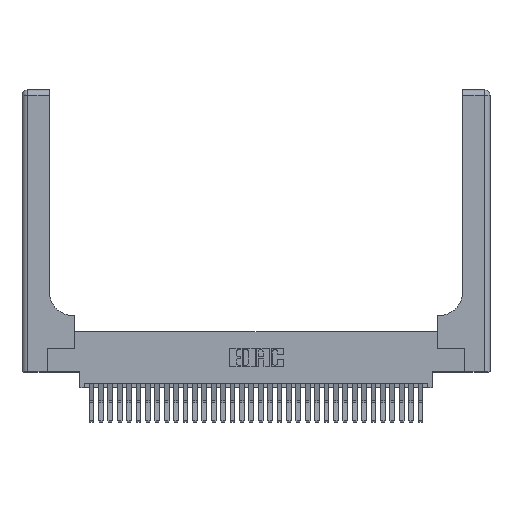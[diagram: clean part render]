
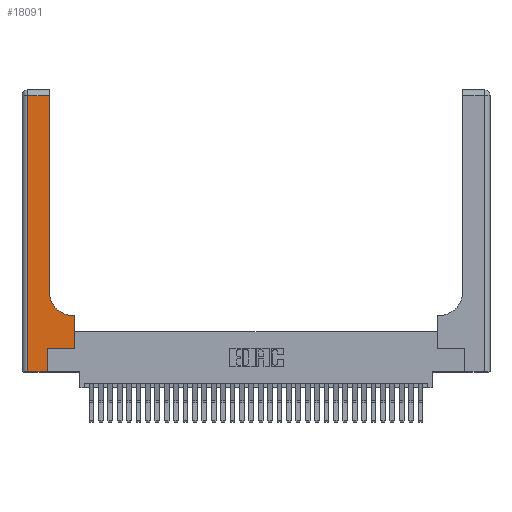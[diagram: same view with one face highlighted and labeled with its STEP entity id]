
A CAD part, top view. The second image highlights one B-rep face of the part: STEP entity #18091.
In plain terms, the highlighted planar face has unit normal (0, 0, 1).
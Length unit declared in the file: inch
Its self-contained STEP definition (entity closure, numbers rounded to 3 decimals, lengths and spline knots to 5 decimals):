
#297 = LINE ( 'NONE', #17229, #12011 ) ;
#355 = LINE ( 'NONE', #4672, #33741 ) ;
#664 = LINE ( 'NONE', #33118, #32364 ) ;
#1186 = VECTOR ( 'NONE', #3302, 39.37008 ) ;
#1492 = DIRECTION ( 'NONE',  ( 0., 1., 0. ) ) ;
#2747 = CARTESIAN_POINT ( 'NONE',  ( 0.2915, 0.6, 0.37 ) ) ;
#2825 = DIRECTION ( 'NONE',  ( -1., 0., 0. ) ) ;
#3302 = DIRECTION ( 'NONE',  ( 1., 0., 0. ) ) ;
#3813 = ORIENTED_EDGE ( 'NONE', *, *, #15643, .T. ) ;
#4265 = DIRECTION ( 'NONE',  ( 0., 1., 0. ) ) ;
#4672 = CARTESIAN_POINT ( 'NONE',  ( 0., 2.94, 0.37 ) ) ;
#4776 = CARTESIAN_POINT ( 'NONE',  ( 0.5585, 0.6, 0.37 ) ) ;
#5122 = EDGE_CURVE ( 'NONE', #22650, #27506, #7500, .T. ) ;
#5214 = ORIENTED_EDGE ( 'NONE', *, *, #11760, .T. ) ;
#5656 = EDGE_CURVE ( 'NONE', #18850, #22650, #297, .T. ) ;
#6736 = VECTOR ( 'NONE', #21437, 39.37008 ) ;
#6989 = DIRECTION ( 'NONE',  ( 0., -1., 0. ) ) ;
#7443 = VERTEX_POINT ( 'NONE', #14530 ) ;
#7500 = LINE ( 'NONE', #32533, #1186 ) ;
#8031 = ORIENTED_EDGE ( 'NONE', *, *, #20928, .T. ) ;
#8523 = VECTOR ( 'NONE', #1492, 39.37008 ) ;
#8974 = CARTESIAN_POINT ( 'NONE',  ( 0., 0., 0.37 ) ) ;
#10153 = CARTESIAN_POINT ( 'NONE',  ( 0.06, 2.94, 0.37 ) ) ;
#10676 = CARTESIAN_POINT ( 'NONE',  ( 0.269, 0., 0.37 ) ) ;
#10985 = CARTESIAN_POINT ( 'NONE',  ( 0., 3., 0.37 ) ) ;
#11760 = EDGE_CURVE ( 'NONE', #7443, #22572, #18933, .T. ) ;
#11864 = VERTEX_POINT ( 'NONE', #4776 ) ;
#12011 = VECTOR ( 'NONE', #4265, 39.37008 ) ;
#12530 = ORIENTED_EDGE ( 'NONE', *, *, #5122, .T. ) ;
#14507 = VERTEX_POINT ( 'NONE', #30355 ) ;
#14530 = CARTESIAN_POINT ( 'NONE',  ( 0.5415, 0.6, 0.37 ) ) ;
#15287 = CARTESIAN_POINT ( 'NONE',  ( 0.5415, 0.85, 0.37 ) ) ;
#15643 = EDGE_CURVE ( 'NONE', #14507, #18850, #26165, .T. ) ;
#15722 = VECTOR ( 'NONE', #6989, 39.37008 ) ;
#15781 = CARTESIAN_POINT ( 'NONE',  ( 0.2915, 0.85, 0.37 ) ) ;
#16157 = ORIENTED_EDGE ( 'NONE', *, *, #5656, .T. ) ;
#16248 = ORIENTED_EDGE ( 'NONE', *, *, #33507, .T. ) ;
#16541 = EDGE_CURVE ( 'NONE', #27506, #11864, #27275, .T. ) ;
#17214 = DIRECTION ( 'NONE',  ( 0., 1., 0. ) ) ;
#17229 = CARTESIAN_POINT ( 'NONE',  ( 0.269, 0., 0.37 ) ) ;
#17428 = VERTEX_POINT ( 'NONE', #10153 ) ;
#17534 = EDGE_LOOP ( 'NONE', ( #8031, #16248, #26795, #3813, #16157, #12530, #29705, #31972, #5214 ) ) ;
#17753 = EDGE_CURVE ( 'NONE', #11864, #7443, #22589, .T. ) ;
#18091 = ADVANCED_FACE ( 'NONE', ( #22554 ), #20956, .F. ) ;
#18543 = DIRECTION ( 'NONE',  ( -1., 0., 0. ) ) ;
#18850 = VERTEX_POINT ( 'NONE', #10676 ) ;
#18933 = CIRCLE ( 'NONE', #20969, 0.25 ) ;
#19139 = DIRECTION ( 'NONE',  ( 0., 0., -1. ) ) ;
#20928 = EDGE_CURVE ( 'NONE', #22572, #26198, #664, .T. ) ;
#20956 = PLANE ( 'NONE',  #27116 ) ;
#20969 = AXIS2_PLACEMENT_3D ( 'NONE', #15287, #26011, #34111 ) ;
#21437 = DIRECTION ( 'NONE',  ( -1., 0., 0. ) ) ;
#22554 = FACE_OUTER_BOUND ( 'NONE', #17534, .T. ) ;
#22572 = VERTEX_POINT ( 'NONE', #15781 ) ;
#22589 = LINE ( 'NONE', #2747, #6736 ) ;
#22650 = VERTEX_POINT ( 'NONE', #33993 ) ;
#24460 = VECTOR ( 'NONE', #30553, 39.37008 ) ;
#25759 = CARTESIAN_POINT ( 'NONE',  ( 0.06, 3., 0.37 ) ) ;
#26011 = DIRECTION ( 'NONE',  ( 0., 0., -1. ) ) ;
#26165 = LINE ( 'NONE', #8974, #24460 ) ;
#26198 = VERTEX_POINT ( 'NONE', #34043 ) ;
#26571 = CARTESIAN_POINT ( 'NONE',  ( 0.5585, 0.25, 0.37 ) ) ;
#26795 = ORIENTED_EDGE ( 'NONE', *, *, #27968, .T. ) ;
#27116 = AXIS2_PLACEMENT_3D ( 'NONE', #10985, #19139, #2825 ) ;
#27275 = LINE ( 'NONE', #33409, #8523 ) ;
#27506 = VERTEX_POINT ( 'NONE', #26571 ) ;
#27968 = EDGE_CURVE ( 'NONE', #17428, #14507, #29854, .T. ) ;
#29705 = ORIENTED_EDGE ( 'NONE', *, *, #16541, .T. ) ;
#29854 = LINE ( 'NONE', #25759, #15722 ) ;
#30355 = CARTESIAN_POINT ( 'NONE',  ( 0.06, 0., 0.37 ) ) ;
#30553 = DIRECTION ( 'NONE',  ( 1., 0., 0. ) ) ;
#31972 = ORIENTED_EDGE ( 'NONE', *, *, #17753, .T. ) ;
#32364 = VECTOR ( 'NONE', #17214, 39.37008 ) ;
#32533 = CARTESIAN_POINT ( 'NONE',  ( 0.269, 0.25, 0.37 ) ) ;
#33118 = CARTESIAN_POINT ( 'NONE',  ( 0.2915, 3., 0.37 ) ) ;
#33409 = CARTESIAN_POINT ( 'NONE',  ( 0.5585, 0.25, 0.37 ) ) ;
#33507 = EDGE_CURVE ( 'NONE', #26198, #17428, #355, .T. ) ;
#33741 = VECTOR ( 'NONE', #18543, 39.37008 ) ;
#33993 = CARTESIAN_POINT ( 'NONE',  ( 0.269, 0.25, 0.37 ) ) ;
#34043 = CARTESIAN_POINT ( 'NONE',  ( 0.2915, 2.94, 0.37 ) ) ;
#34111 = DIRECTION ( 'NONE',  ( 1., 0., 0. ) ) ;
